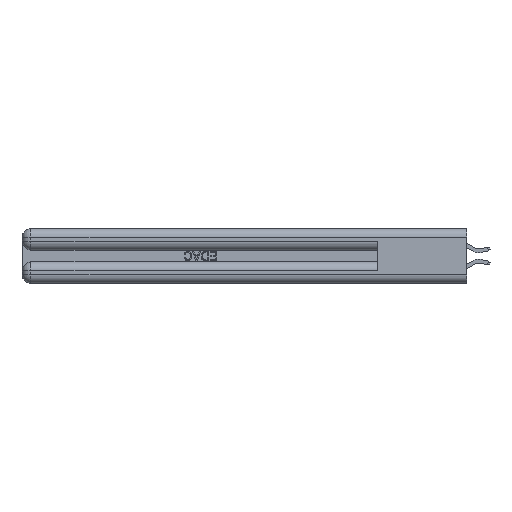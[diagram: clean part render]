
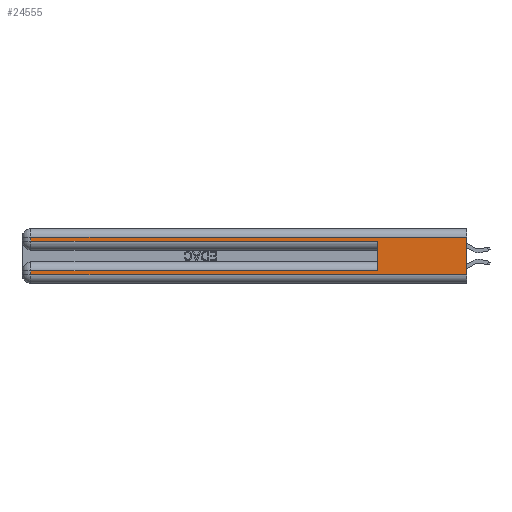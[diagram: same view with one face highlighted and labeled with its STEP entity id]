
A CAD part, left-side view. The second image highlights one B-rep face of the part: STEP entity #24555.
In plain terms, the highlighted planar face has unit normal (-1, 0, 0).
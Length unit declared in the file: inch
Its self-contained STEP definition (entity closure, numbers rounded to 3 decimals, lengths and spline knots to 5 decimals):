
#399 = CARTESIAN_POINT ( 'NONE',  ( 0., 2.94, 0.31 ) ) ;
#958 = DIRECTION ( 'NONE',  ( 0., 1., 0. ) ) ;
#1057 = AXIS2_PLACEMENT_3D ( 'NONE', #28258, #24704, #28409 ) ;
#1198 = VERTEX_POINT ( 'NONE', #26267 ) ;
#3494 = VECTOR ( 'NONE', #43065, 39.37008 ) ;
#4193 = EDGE_CURVE ( 'NONE', #36303, #1198, #38778, .T. ) ;
#5585 = ORIENTED_EDGE ( 'NONE', *, *, #4193, .T. ) ;
#6163 = ORIENTED_EDGE ( 'NONE', *, *, #31344, .T. ) ;
#7908 = CARTESIAN_POINT ( 'NONE',  ( 0., 2.94, 0.06 ) ) ;
#8156 = LINE ( 'NONE', #23214, #9916 ) ;
#8851 = DIRECTION ( 'NONE',  ( 0., 0., -1. ) ) ;
#9048 = EDGE_CURVE ( 'NONE', #25055, #13603, #28905, .T. ) ;
#9916 = VECTOR ( 'NONE', #11979, 39.37008 ) ;
#11804 = FACE_OUTER_BOUND ( 'NONE', #13254, .T. ) ;
#11979 = DIRECTION ( 'NONE',  ( 0., -1., 0. ) ) ;
#12382 = CARTESIAN_POINT ( 'NONE',  ( 0., 0., 0.06 ) ) ;
#12528 = CARTESIAN_POINT ( 'NONE',  ( 0., 0.6, 0.145 ) ) ;
#12855 = LINE ( 'NONE', #39239, #18553 ) ;
#13059 = VECTOR ( 'NONE', #45165, 39.37008 ) ;
#13254 = EDGE_LOOP ( 'NONE', ( #46276, #6163, #5585, #44892, #35864, #24346, #25099, #22956 ) ) ;
#13603 = VERTEX_POINT ( 'NONE', #28386 ) ;
#13759 = EDGE_CURVE ( 'NONE', #43504, #19427, #32667, .T. ) ;
#15605 = CARTESIAN_POINT ( 'NONE',  ( 0., 0., 0.085 ) ) ;
#15890 = CARTESIAN_POINT ( 'NONE',  ( 0., 2.94, 0.085 ) ) ;
#16975 = CARTESIAN_POINT ( 'NONE',  ( 0., 0., 0.31 ) ) ;
#18553 = VECTOR ( 'NONE', #32039, 39.37008 ) ;
#19090 = EDGE_CURVE ( 'NONE', #1198, #13603, #8156, .T. ) ;
#19380 = CARTESIAN_POINT ( 'NONE',  ( 0., 0., 0.37 ) ) ;
#19427 = VERTEX_POINT ( 'NONE', #12382 ) ;
#19694 = DIRECTION ( 'NONE',  ( 0., 0., -1. ) ) ;
#20100 = LINE ( 'NONE', #31702, #3494 ) ;
#20639 = LINE ( 'NONE', #15605, #37157 ) ;
#21285 = VECTOR ( 'NONE', #8851, 39.37008 ) ;
#21748 = VERTEX_POINT ( 'NONE', #7908 ) ;
#22956 = ORIENTED_EDGE ( 'NONE', *, *, #29181, .T. ) ;
#23214 = CARTESIAN_POINT ( 'NONE',  ( 0., 0., 0.285 ) ) ;
#24346 = ORIENTED_EDGE ( 'NONE', *, *, #29699, .T. ) ;
#24555 = ADVANCED_FACE ( 'NONE', ( #11804 ), #34595, .F. ) ;
#24704 = DIRECTION ( 'NONE',  ( 1., 0., 0. ) ) ;
#25055 = VERTEX_POINT ( 'NONE', #33308 ) ;
#25099 = ORIENTED_EDGE ( 'NONE', *, *, #26821, .T. ) ;
#25274 = VERTEX_POINT ( 'NONE', #15890 ) ;
#26267 = CARTESIAN_POINT ( 'NONE',  ( 0., 2.94, 0.285 ) ) ;
#26821 = EDGE_CURVE ( 'NONE', #25274, #21748, #12855, .T. ) ;
#27962 = LINE ( 'NONE', #38055, #13059 ) ;
#28258 = CARTESIAN_POINT ( 'NONE',  ( 0., 0., 0.37 ) ) ;
#28386 = CARTESIAN_POINT ( 'NONE',  ( 0., 0.6, 0.285 ) ) ;
#28409 = DIRECTION ( 'NONE',  ( 0., 0., -1. ) ) ;
#28905 = LINE ( 'NONE', #12528, #39718 ) ;
#29181 = EDGE_CURVE ( 'NONE', #21748, #19427, #20100, .T. ) ;
#29699 = EDGE_CURVE ( 'NONE', #25055, #25274, #20639, .T. ) ;
#30428 = CARTESIAN_POINT ( 'NONE',  ( 0., 2.94, 0.37 ) ) ;
#31344 = EDGE_CURVE ( 'NONE', #43504, #36303, #27962, .T. ) ;
#31702 = CARTESIAN_POINT ( 'NONE',  ( 0., 0., 0.06 ) ) ;
#32039 = DIRECTION ( 'NONE',  ( 0., 0., -1. ) ) ;
#32667 = LINE ( 'NONE', #19380, #21285 ) ;
#33308 = CARTESIAN_POINT ( 'NONE',  ( 0., 0.6, 0.085 ) ) ;
#34069 = DIRECTION ( 'NONE',  ( 0., 0., 1. ) ) ;
#34595 = PLANE ( 'NONE',  #1057 ) ;
#35864 = ORIENTED_EDGE ( 'NONE', *, *, #9048, .F. ) ;
#36303 = VERTEX_POINT ( 'NONE', #399 ) ;
#37157 = VECTOR ( 'NONE', #958, 39.37008 ) ;
#38055 = CARTESIAN_POINT ( 'NONE',  ( 0., 0., 0.31 ) ) ;
#38778 = LINE ( 'NONE', #30428, #44540 ) ;
#39239 = CARTESIAN_POINT ( 'NONE',  ( 0., 2.94, 0.37 ) ) ;
#39718 = VECTOR ( 'NONE', #34069, 39.37008 ) ;
#43065 = DIRECTION ( 'NONE',  ( 0., -1., 0. ) ) ;
#43504 = VERTEX_POINT ( 'NONE', #16975 ) ;
#44540 = VECTOR ( 'NONE', #19694, 39.37008 ) ;
#44892 = ORIENTED_EDGE ( 'NONE', *, *, #19090, .T. ) ;
#45165 = DIRECTION ( 'NONE',  ( 0., 1., 0. ) ) ;
#46276 = ORIENTED_EDGE ( 'NONE', *, *, #13759, .F. ) ;
